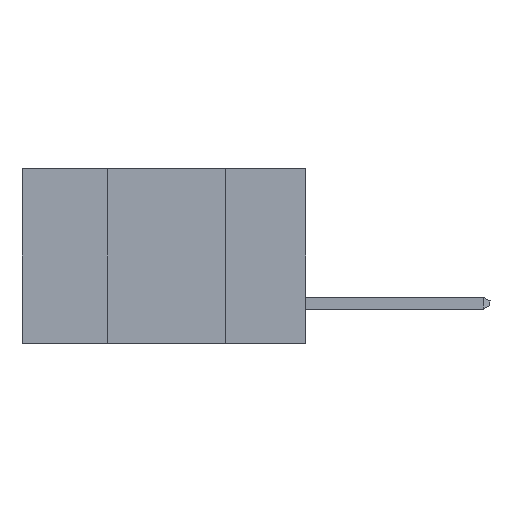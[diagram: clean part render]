
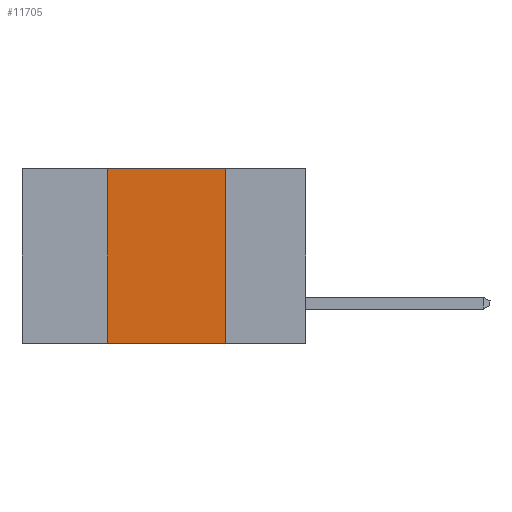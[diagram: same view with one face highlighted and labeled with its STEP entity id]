
A CAD part, left-side view. The second image highlights one B-rep face of the part: STEP entity #11705.
In plain terms, the highlighted planar face has unit normal (-1, 0, 0).
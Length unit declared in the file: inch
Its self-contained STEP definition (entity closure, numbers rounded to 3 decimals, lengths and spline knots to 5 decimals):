
#292 = DIRECTION ( 'NONE',  ( 1., 0., 0. ) ) ;
#379 = FACE_OUTER_BOUND ( 'NONE', #1310, .T. ) ;
#1310 = EDGE_LOOP ( 'NONE', ( #15817, #4122, #16212, #9392 ) ) ;
#4122 = ORIENTED_EDGE ( 'NONE', *, *, #10946, .F. ) ;
#4343 = VERTEX_POINT ( 'NONE', #13336 ) ;
#4627 = PLANE ( 'NONE',  #17432 ) ;
#5349 = VECTOR ( 'NONE', #17322, 39.37008 ) ;
#5520 = CARTESIAN_POINT ( 'NONE',  ( 0., 0.17, -0.37 ) ) ;
#5616 = DIRECTION ( 'NONE',  ( 0., 0., -1. ) ) ;
#6062 = CARTESIAN_POINT ( 'NONE',  ( 0., 0.6, 0. ) ) ;
#7452 = DIRECTION ( 'NONE',  ( 0., 0., -1. ) ) ;
#8230 = CARTESIAN_POINT ( 'NONE',  ( 0., 0.6, 0. ) ) ;
#8421 = LINE ( 'NONE', #8230, #5349 ) ;
#8676 = CARTESIAN_POINT ( 'NONE',  ( 0., 0.42, 0. ) ) ;
#9082 = DIRECTION ( 'NONE',  ( 0., 0., 1. ) ) ;
#9392 = ORIENTED_EDGE ( 'NONE', *, *, #17987, .T. ) ;
#9540 = CARTESIAN_POINT ( 'NONE',  ( 0., 0.17, 0. ) ) ;
#10712 = CARTESIAN_POINT ( 'NONE',  ( 0., 0.42, -0.37 ) ) ;
#10946 = EDGE_CURVE ( 'NONE', #17893, #18527, #8421, .T. ) ;
#11191 = EDGE_CURVE ( 'NONE', #15877, #17893, #13450, .T. ) ;
#11705 = ADVANCED_FACE ( 'NONE', ( #379 ), #4627, .F. ) ;
#12034 = LINE ( 'NONE', #12318, #15419 ) ;
#12318 = CARTESIAN_POINT ( 'NONE',  ( 0., 0.6, -0.37 ) ) ;
#13336 = CARTESIAN_POINT ( 'NONE',  ( 0., 0.17, -0.37 ) ) ;
#13450 = LINE ( 'NONE', #10712, #18330 ) ;
#15419 = VECTOR ( 'NONE', #17934, 39.37008 ) ;
#15817 = ORIENTED_EDGE ( 'NONE', *, *, #19009, .F. ) ;
#15877 = VERTEX_POINT ( 'NONE', #16758 ) ;
#16071 = VECTOR ( 'NONE', #5616, 39.37008 ) ;
#16212 = ORIENTED_EDGE ( 'NONE', *, *, #11191, .F. ) ;
#16758 = CARTESIAN_POINT ( 'NONE',  ( 0., 0.42, -0.37 ) ) ;
#17322 = DIRECTION ( 'NONE',  ( 0., -1., 0. ) ) ;
#17432 = AXIS2_PLACEMENT_3D ( 'NONE', #6062, #292, #7452 ) ;
#17893 = VERTEX_POINT ( 'NONE', #8676 ) ;
#17934 = DIRECTION ( 'NONE',  ( 0., -1., 0. ) ) ;
#17987 = EDGE_CURVE ( 'NONE', #15877, #4343, #12034, .T. ) ;
#18330 = VECTOR ( 'NONE', #9082, 39.37008 ) ;
#18527 = VERTEX_POINT ( 'NONE', #9540 ) ;
#18879 = LINE ( 'NONE', #5520, #16071 ) ;
#19009 = EDGE_CURVE ( 'NONE', #18527, #4343, #18879, .T. ) ;
